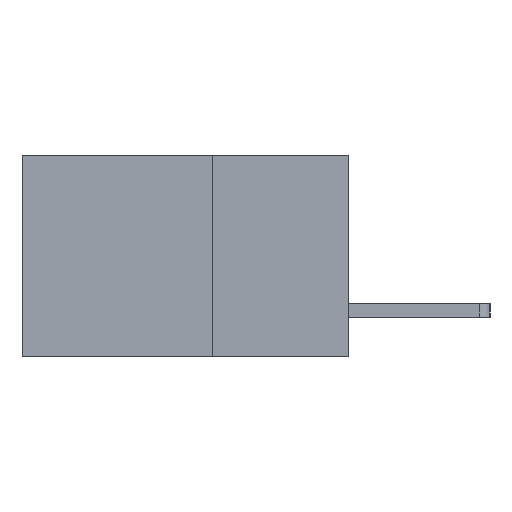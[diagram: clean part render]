
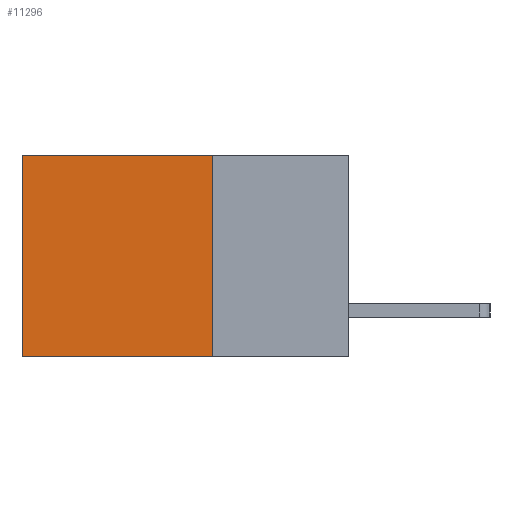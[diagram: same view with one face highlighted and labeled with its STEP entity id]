
A CAD part, left-side view. The second image highlights one B-rep face of the part: STEP entity #11296.
In plain terms, the highlighted planar face has unit normal (-1, 0, 0).
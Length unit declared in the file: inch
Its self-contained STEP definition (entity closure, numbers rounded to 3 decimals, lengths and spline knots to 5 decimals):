
#105 = CARTESIAN_POINT ( 'NONE',  ( 0.298, 0.25, -0.37 ) ) ;
#260 = LINE ( 'NONE', #4787, #4810 ) ;
#295 = DIRECTION ( 'NONE',  ( 0., 0., -1. ) ) ;
#511 = VERTEX_POINT ( 'NONE', #105 ) ;
#602 = FACE_OUTER_BOUND ( 'NONE', #3625, .T. ) ;
#622 = CARTESIAN_POINT ( 'NONE',  ( 0.298, 0.25, 0. ) ) ;
#1080 = EDGE_CURVE ( 'NONE', #1753, #6803, #5097, .T. ) ;
#1177 = EDGE_CURVE ( 'NONE', #1753, #511, #6378, .T. ) ;
#1306 = ORIENTED_EDGE ( 'NONE', *, *, #1080, .T. ) ;
#1523 = DIRECTION ( 'NONE',  ( 1., 0., 0. ) ) ;
#1753 = VERTEX_POINT ( 'NONE', #5470 ) ;
#2215 = ORIENTED_EDGE ( 'NONE', *, *, #1177, .F. ) ;
#2283 = EDGE_CURVE ( 'NONE', #6803, #9288, #260, .T. ) ;
#2654 = VECTOR ( 'NONE', #6721, 39.37008 ) ;
#2773 = CARTESIAN_POINT ( 'NONE',  ( 0.298, 0.6, -0.37 ) ) ;
#3625 = EDGE_LOOP ( 'NONE', ( #8365, #4922, #2215, #1306 ) ) ;
#3662 = EDGE_CURVE ( 'NONE', #511, #9288, #4493, .T. ) ;
#4493 = LINE ( 'NONE', #6253, #8974 ) ;
#4787 = CARTESIAN_POINT ( 'NONE',  ( 0.298, 0.6, 0. ) ) ;
#4810 = VECTOR ( 'NONE', #295, 39.37008 ) ;
#4922 = ORIENTED_EDGE ( 'NONE', *, *, #3662, .F. ) ;
#5097 = LINE ( 'NONE', #8618, #2654 ) ;
#5470 = CARTESIAN_POINT ( 'NONE',  ( 0.298, 0.25, 0. ) ) ;
#5981 = DIRECTION ( 'NONE',  ( 0., 0., -1. ) ) ;
#6253 = CARTESIAN_POINT ( 'NONE',  ( 0.298, 0.25, -0.37 ) ) ;
#6378 = LINE ( 'NONE', #8229, #8989 ) ;
#6721 = DIRECTION ( 'NONE',  ( 0., 1., 0. ) ) ;
#6803 = VERTEX_POINT ( 'NONE', #8853 ) ;
#6985 = PLANE ( 'NONE',  #7816 ) ;
#7816 = AXIS2_PLACEMENT_3D ( 'NONE', #622, #1523, #7874 ) ;
#7874 = DIRECTION ( 'NONE',  ( 0., 0., -1. ) ) ;
#8229 = CARTESIAN_POINT ( 'NONE',  ( 0.298, 0.25, 0. ) ) ;
#8365 = ORIENTED_EDGE ( 'NONE', *, *, #2283, .T. ) ;
#8618 = CARTESIAN_POINT ( 'NONE',  ( 0.298, 0.25, 0. ) ) ;
#8853 = CARTESIAN_POINT ( 'NONE',  ( 0.298, 0.6, 0. ) ) ;
#8928 = DIRECTION ( 'NONE',  ( 0., 1., 0. ) ) ;
#8974 = VECTOR ( 'NONE', #8928, 39.37008 ) ;
#8989 = VECTOR ( 'NONE', #5981, 39.37008 ) ;
#9288 = VERTEX_POINT ( 'NONE', #2773 ) ;
#11296 = ADVANCED_FACE ( 'NONE', ( #602 ), #6985, .F. ) ;
